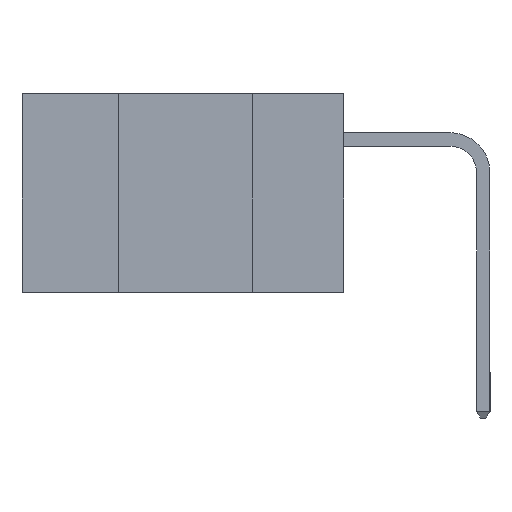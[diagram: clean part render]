
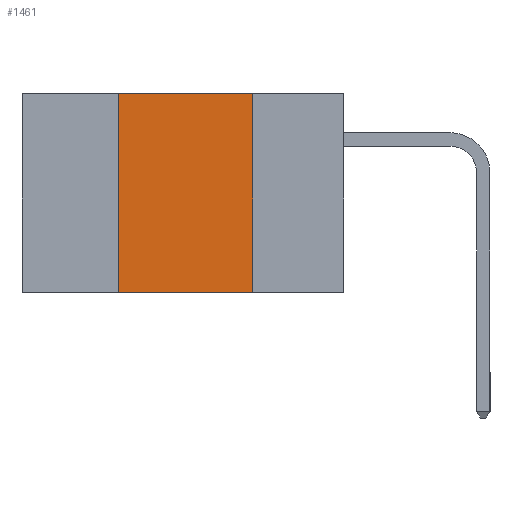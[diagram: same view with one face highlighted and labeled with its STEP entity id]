
A CAD part, left-side view. The second image highlights one B-rep face of the part: STEP entity #1461.
In plain terms, the highlighted planar face has unit normal (-1, 0, 0).
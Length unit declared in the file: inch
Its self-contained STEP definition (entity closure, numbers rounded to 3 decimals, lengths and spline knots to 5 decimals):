
#45 = CARTESIAN_POINT ( 'NONE',  ( 0., 0.6, -0.37 ) ) ;
#251 = ORIENTED_EDGE ( 'NONE', *, *, #2120, .T. ) ;
#1200 = VECTOR ( 'NONE', #10845, 39.37008 ) ;
#1461 = ADVANCED_FACE ( 'NONE', ( #7309 ), #7259, .F. ) ;
#2120 = EDGE_CURVE ( 'NONE', #10480, #8068, #8133, .T. ) ;
#2559 = VERTEX_POINT ( 'NONE', #7410 ) ;
#2720 = CARTESIAN_POINT ( 'NONE',  ( 0., 0.6, 0. ) ) ;
#2859 = EDGE_LOOP ( 'NONE', ( #4679, #8480, #10748, #251 ) ) ;
#3167 = EDGE_CURVE ( 'NONE', #10480, #2559, #11518, .T. ) ;
#3256 = EDGE_CURVE ( 'NONE', #2559, #4036, #8248, .T. ) ;
#3270 = AXIS2_PLACEMENT_3D ( 'NONE', #2720, #10099, #8090 ) ;
#3431 = CARTESIAN_POINT ( 'NONE',  ( 0., 0.42, -0.37 ) ) ;
#3493 = DIRECTION ( 'NONE',  ( 0., 0., 1. ) ) ;
#3514 = DIRECTION ( 'NONE',  ( 0., 0., -1. ) ) ;
#4036 = VERTEX_POINT ( 'NONE', #5350 ) ;
#4679 = ORIENTED_EDGE ( 'NONE', *, *, #7464, .F. ) ;
#5345 = VECTOR ( 'NONE', #10730, 39.37008 ) ;
#5350 = CARTESIAN_POINT ( 'NONE',  ( 0., 0.17, 0. ) ) ;
#5509 = CARTESIAN_POINT ( 'NONE',  ( 0., 0.17, -0.37 ) ) ;
#6955 = VECTOR ( 'NONE', #3514, 39.37008 ) ;
#7259 = PLANE ( 'NONE',  #3270 ) ;
#7309 = FACE_OUTER_BOUND ( 'NONE', #2859, .T. ) ;
#7410 = CARTESIAN_POINT ( 'NONE',  ( 0., 0.42, 0. ) ) ;
#7464 = EDGE_CURVE ( 'NONE', #4036, #8068, #8049, .T. ) ;
#7550 = CARTESIAN_POINT ( 'NONE',  ( 0., 0.17, -0.37 ) ) ;
#8049 = LINE ( 'NONE', #5509, #6955 ) ;
#8068 = VERTEX_POINT ( 'NONE', #7550 ) ;
#8090 = DIRECTION ( 'NONE',  ( 0., 0., -1. ) ) ;
#8133 = LINE ( 'NONE', #45, #1200 ) ;
#8135 = CARTESIAN_POINT ( 'NONE',  ( 0., 0.6, 0. ) ) ;
#8248 = LINE ( 'NONE', #8135, #5345 ) ;
#8480 = ORIENTED_EDGE ( 'NONE', *, *, #3256, .F. ) ;
#9301 = CARTESIAN_POINT ( 'NONE',  ( 0., 0.42, -0.37 ) ) ;
#9311 = VECTOR ( 'NONE', #3493, 39.37008 ) ;
#10099 = DIRECTION ( 'NONE',  ( 1., 0., 0. ) ) ;
#10480 = VERTEX_POINT ( 'NONE', #9301 ) ;
#10730 = DIRECTION ( 'NONE',  ( 0., -1., 0. ) ) ;
#10748 = ORIENTED_EDGE ( 'NONE', *, *, #3167, .F. ) ;
#10845 = DIRECTION ( 'NONE',  ( 0., -1., 0. ) ) ;
#11518 = LINE ( 'NONE', #3431, #9311 ) ;
